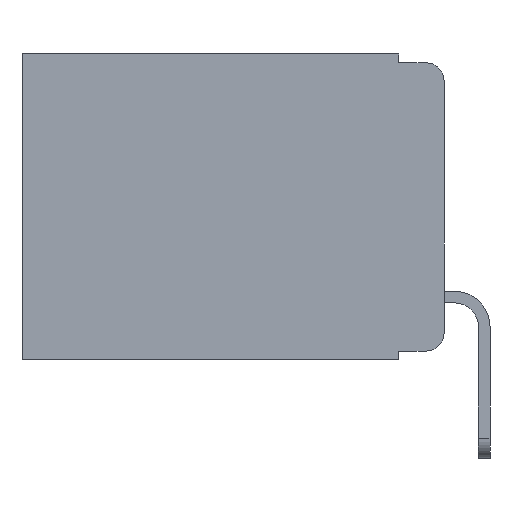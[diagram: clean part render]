
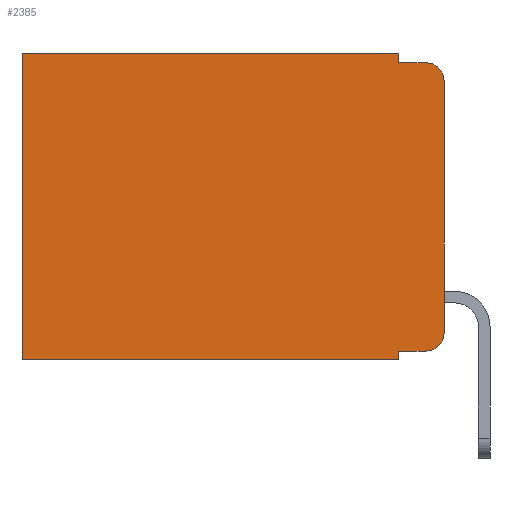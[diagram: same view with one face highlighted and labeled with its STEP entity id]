
A CAD part, left-side view. The second image highlights one B-rep face of the part: STEP entity #2385.
In plain terms, the highlighted planar face has unit normal (-1, 0, 0).
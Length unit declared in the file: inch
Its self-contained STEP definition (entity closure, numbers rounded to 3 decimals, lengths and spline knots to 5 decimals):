
#120 = LINE ( 'NONE', #5937, #2539 ) ;
#275 = CARTESIAN_POINT ( 'NONE',  ( 0.298, 0., -0.313 ) ) ;
#463 = DIRECTION ( 'NONE',  ( 0., 1., 0. ) ) ;
#545 = VERTEX_POINT ( 'NONE', #9482 ) ;
#768 = VERTEX_POINT ( 'NONE', #4533 ) ;
#813 = VERTEX_POINT ( 'NONE', #2699 ) ;
#834 = ORIENTED_EDGE ( 'NONE', *, *, #8688, .F. ) ;
#1190 = CARTESIAN_POINT ( 'NONE',  ( 0.298, 0., -0.343 ) ) ;
#1534 = ORIENTED_EDGE ( 'NONE', *, *, #2751, .T. ) ;
#1821 = AXIS2_PLACEMENT_3D ( 'NONE', #8172, #7756, #7593 ) ;
#2016 = ORIENTED_EDGE ( 'NONE', *, *, #2731, .T. ) ;
#2081 = CARTESIAN_POINT ( 'NONE',  ( 0.298, 0., 0. ) ) ;
#2385 = ADVANCED_FACE ( 'NONE', ( #6899 ), #4518, .F. ) ;
#2497 = LINE ( 'NONE', #1190, #4304 ) ;
#2505 = EDGE_CURVE ( 'NONE', #813, #8614, #3287, .T. ) ;
#2539 = VECTOR ( 'NONE', #9943, 39.37008 ) ;
#2563 = EDGE_CURVE ( 'NONE', #4150, #768, #6376, .T. ) ;
#2584 = EDGE_CURVE ( 'NONE', #813, #5777, #3968, .T. ) ;
#2629 = EDGE_CURVE ( 'NONE', #545, #5777, #3147, .T. ) ;
#2653 = EDGE_CURVE ( 'NONE', #4150, #545, #120, .T. ) ;
#2699 = CARTESIAN_POINT ( 'NONE',  ( 0.298, 0., -0.03 ) ) ;
#2731 = EDGE_CURVE ( 'NONE', #768, #5646, #9428, .T. ) ;
#2734 = EDGE_CURVE ( 'NONE', #2843, #6684, #5161, .T. ) ;
#2737 = EDGE_CURVE ( 'NONE', #2843, #5039, #6937, .T. ) ;
#2751 = EDGE_CURVE ( 'NONE', #5039, #8614, #10114, .T. ) ;
#2843 = VERTEX_POINT ( 'NONE', #3456 ) ;
#2851 = DIRECTION ( 'NONE',  ( 0., 1., 0. ) ) ;
#2924 = ORIENTED_EDGE ( 'NONE', *, *, #2505, .F. ) ;
#2951 = VECTOR ( 'NONE', #7129, 39.37008 ) ;
#3147 = LINE ( 'NONE', #4961, #3441 ) ;
#3193 = DIRECTION ( 'NONE',  ( 0., -1., 0. ) ) ;
#3287 = LINE ( 'NONE', #7881, #6800 ) ;
#3441 = VECTOR ( 'NONE', #3193, 39.37008 ) ;
#3456 = CARTESIAN_POINT ( 'NONE',  ( 0.298, 0.051, -0.333 ) ) ;
#3689 = ORIENTED_EDGE ( 'NONE', *, *, #2629, .F. ) ;
#3968 = CIRCLE ( 'NONE', #1821, 0.02 ) ;
#4150 = VERTEX_POINT ( 'NONE', #9529 ) ;
#4304 = VECTOR ( 'NONE', #2851, 39.37008 ) ;
#4518 = PLANE ( 'NONE',  #8641 ) ;
#4533 = CARTESIAN_POINT ( 'NONE',  ( 0.298, 0.473, 0. ) ) ;
#4700 = EDGE_LOOP ( 'NONE', ( #2924, #8711, #3689, #7517, #8774, #2016, #834, #8871, #8676, #1534 ) ) ;
#4842 = CARTESIAN_POINT ( 'NONE',  ( 0.298, 0.051, -0.343 ) ) ;
#4889 = CARTESIAN_POINT ( 'NONE',  ( 0.298, 0.051, 0. ) ) ;
#4961 = CARTESIAN_POINT ( 'NONE',  ( 0.298, 0.051, -0.01 ) ) ;
#5039 = VERTEX_POINT ( 'NONE', #9504 ) ;
#5161 = LINE ( 'NONE', #4889, #2951 ) ;
#5646 = VERTEX_POINT ( 'NONE', #7393 ) ;
#5698 = DIRECTION ( 'NONE',  ( 1., 0., 0. ) ) ;
#5725 = DIRECTION ( 'NONE',  ( 0., 0., -1. ) ) ;
#5777 = VERTEX_POINT ( 'NONE', #6538 ) ;
#5937 = CARTESIAN_POINT ( 'NONE',  ( 0.298, 0.051, 0. ) ) ;
#5979 = DIRECTION ( 'NONE',  ( 0., 0., -1. ) ) ;
#6191 = VECTOR ( 'NONE', #463, 39.37008 ) ;
#6376 = LINE ( 'NONE', #6881, #6191 ) ;
#6538 = CARTESIAN_POINT ( 'NONE',  ( 0.298, 0.02, -0.01 ) ) ;
#6684 = VERTEX_POINT ( 'NONE', #4842 ) ;
#6800 = VECTOR ( 'NONE', #8847, 39.37008 ) ;
#6848 = DIRECTION ( 'NONE',  ( -1., 0., 0. ) ) ;
#6881 = CARTESIAN_POINT ( 'NONE',  ( 0.298, 0., 0. ) ) ;
#6882 = CARTESIAN_POINT ( 'NONE',  ( 0.298, 0.02, -0.313 ) ) ;
#6899 = FACE_OUTER_BOUND ( 'NONE', #4700, .T. ) ;
#6937 = LINE ( 'NONE', #7119, #8541 ) ;
#7119 = CARTESIAN_POINT ( 'NONE',  ( 0.298, 0.051, -0.333 ) ) ;
#7129 = DIRECTION ( 'NONE',  ( 0., 0., -1. ) ) ;
#7393 = CARTESIAN_POINT ( 'NONE',  ( 0.298, 0.473, -0.343 ) ) ;
#7400 = DIRECTION ( 'NONE',  ( 0., -1., 0. ) ) ;
#7517 = ORIENTED_EDGE ( 'NONE', *, *, #2653, .F. ) ;
#7593 = DIRECTION ( 'NONE',  ( 0., 0., -1. ) ) ;
#7756 = DIRECTION ( 'NONE',  ( -1., 0., 0. ) ) ;
#7881 = CARTESIAN_POINT ( 'NONE',  ( 0.298, 0., 0. ) ) ;
#8172 = CARTESIAN_POINT ( 'NONE',  ( 0.298, 0.02, -0.03 ) ) ;
#8541 = VECTOR ( 'NONE', #7400, 39.37008 ) ;
#8614 = VERTEX_POINT ( 'NONE', #275 ) ;
#8641 = AXIS2_PLACEMENT_3D ( 'NONE', #2081, #5698, #5725 ) ;
#8676 = ORIENTED_EDGE ( 'NONE', *, *, #2737, .T. ) ;
#8688 = EDGE_CURVE ( 'NONE', #6684, #5646, #2497, .T. ) ;
#8711 = ORIENTED_EDGE ( 'NONE', *, *, #2584, .T. ) ;
#8742 = VECTOR ( 'NONE', #5979, 39.37008 ) ;
#8774 = ORIENTED_EDGE ( 'NONE', *, *, #2563, .T. ) ;
#8793 = CARTESIAN_POINT ( 'NONE',  ( 0.298, 0.473, 0. ) ) ;
#8847 = DIRECTION ( 'NONE',  ( 0., 0., -1. ) ) ;
#8871 = ORIENTED_EDGE ( 'NONE', *, *, #2734, .F. ) ;
#9041 = AXIS2_PLACEMENT_3D ( 'NONE', #6882, #6848, #9884 ) ;
#9428 = LINE ( 'NONE', #8793, #8742 ) ;
#9482 = CARTESIAN_POINT ( 'NONE',  ( 0.298, 0.051, -0.01 ) ) ;
#9504 = CARTESIAN_POINT ( 'NONE',  ( 0.298, 0.02, -0.333 ) ) ;
#9529 = CARTESIAN_POINT ( 'NONE',  ( 0.298, 0.051, 0. ) ) ;
#9884 = DIRECTION ( 'NONE',  ( 0., 0., -1. ) ) ;
#9943 = DIRECTION ( 'NONE',  ( 0., 0., -1. ) ) ;
#10114 = CIRCLE ( 'NONE', #9041, 0.02 ) ;
